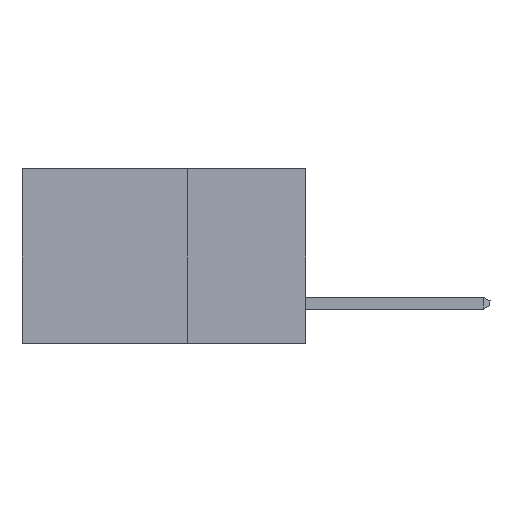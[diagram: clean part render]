
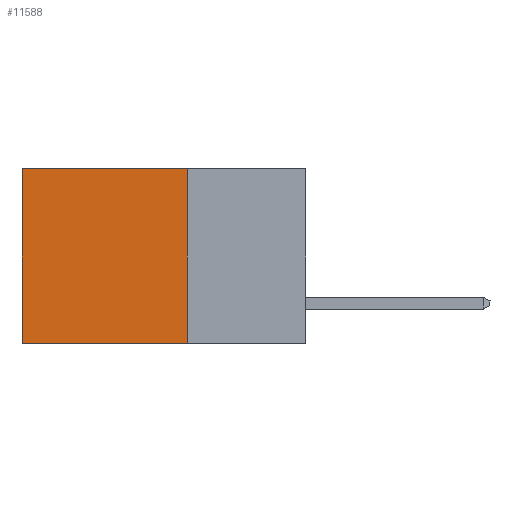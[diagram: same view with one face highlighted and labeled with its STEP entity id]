
A CAD part, left-side view. The second image highlights one B-rep face of the part: STEP entity #11588.
In plain terms, the highlighted planar face has unit normal (-1, 0, 0).
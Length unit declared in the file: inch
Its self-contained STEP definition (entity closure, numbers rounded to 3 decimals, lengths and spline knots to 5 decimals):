
#259 = CARTESIAN_POINT ( 'NONE',  ( 0.2615, 0.6, -0.37 ) ) ;
#376 = VECTOR ( 'NONE', #9385, 39.37008 ) ;
#474 = EDGE_CURVE ( 'NONE', #15411, #6366, #16025, .T. ) ;
#982 = ORIENTED_EDGE ( 'NONE', *, *, #9360, .T. ) ;
#1415 = FACE_OUTER_BOUND ( 'NONE', #11645, .T. ) ;
#2564 = AXIS2_PLACEMENT_3D ( 'NONE', #7881, #11252, #8615 ) ;
#3556 = CARTESIAN_POINT ( 'NONE',  ( 0.2615, 0.25, -0.37 ) ) ;
#3786 = VECTOR ( 'NONE', #19942, 39.37008 ) ;
#4134 = ORIENTED_EDGE ( 'NONE', *, *, #14797, .F. ) ;
#4723 = CARTESIAN_POINT ( 'NONE',  ( 0.2615, 0.25, 0. ) ) ;
#6366 = VERTEX_POINT ( 'NONE', #9637 ) ;
#6372 = DIRECTION ( 'NONE',  ( 0., 0., -1. ) ) ;
#6394 = PLANE ( 'NONE',  #2564 ) ;
#6449 = LINE ( 'NONE', #11084, #12640 ) ;
#6499 = VERTEX_POINT ( 'NONE', #10259 ) ;
#7787 = VECTOR ( 'NONE', #6372, 39.37008 ) ;
#7881 = CARTESIAN_POINT ( 'NONE',  ( 0.2615, 0.25, -0.37 ) ) ;
#8615 = DIRECTION ( 'NONE',  ( 0., 0., -1. ) ) ;
#9339 = CARTESIAN_POINT ( 'NONE',  ( 0.2615, 0.25, -0.37 ) ) ;
#9360 = EDGE_CURVE ( 'NONE', #6366, #19877, #6449, .T. ) ;
#9385 = DIRECTION ( 'NONE',  ( 0., 1., 0. ) ) ;
#9637 = CARTESIAN_POINT ( 'NONE',  ( 0.2615, 0.6, 0. ) ) ;
#10259 = CARTESIAN_POINT ( 'NONE',  ( 0.2615, 0.25, -0.37 ) ) ;
#11084 = CARTESIAN_POINT ( 'NONE',  ( 0.2615, 0.6, -0.37 ) ) ;
#11252 = DIRECTION ( 'NONE',  ( 1., 0., 0. ) ) ;
#11588 = ADVANCED_FACE ( 'NONE', ( #1415 ), #6394, .F. ) ;
#11645 = EDGE_LOOP ( 'NONE', ( #982, #4134, #17379, #20317 ) ) ;
#12640 = VECTOR ( 'NONE', #16145, 39.37008 ) ;
#13285 = EDGE_CURVE ( 'NONE', #15411, #6499, #14391, .T. ) ;
#14391 = LINE ( 'NONE', #9339, #7787 ) ;
#14797 = EDGE_CURVE ( 'NONE', #6499, #19877, #15171, .T. ) ;
#15171 = LINE ( 'NONE', #3556, #3786 ) ;
#15411 = VERTEX_POINT ( 'NONE', #18737 ) ;
#16025 = LINE ( 'NONE', #4723, #376 ) ;
#16145 = DIRECTION ( 'NONE',  ( 0., 0., -1. ) ) ;
#17379 = ORIENTED_EDGE ( 'NONE', *, *, #13285, .F. ) ;
#18737 = CARTESIAN_POINT ( 'NONE',  ( 0.2615, 0.25, 0. ) ) ;
#19877 = VERTEX_POINT ( 'NONE', #259 ) ;
#19942 = DIRECTION ( 'NONE',  ( 0., 1., 0. ) ) ;
#20317 = ORIENTED_EDGE ( 'NONE', *, *, #474, .T. ) ;
